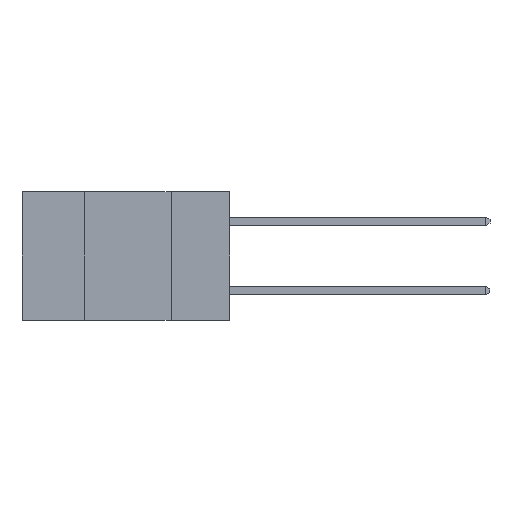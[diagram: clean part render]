
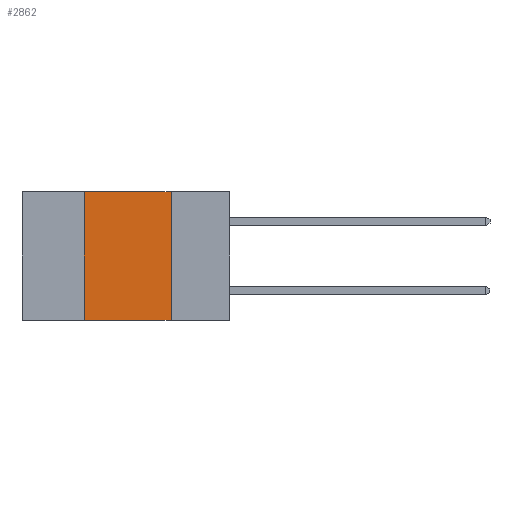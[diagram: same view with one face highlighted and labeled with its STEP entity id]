
A CAD part, left-side view. The second image highlights one B-rep face of the part: STEP entity #2862.
In plain terms, the highlighted planar face has unit normal (-1, 0, 0).
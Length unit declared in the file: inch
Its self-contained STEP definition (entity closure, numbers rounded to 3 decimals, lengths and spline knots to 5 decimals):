
#152 = CARTESIAN_POINT ( 'NONE',  ( 0., 0.42, -0.37 ) ) ;
#434 = AXIS2_PLACEMENT_3D ( 'NONE', #6717, #8320, #8428 ) ;
#1531 = CARTESIAN_POINT ( 'NONE',  ( 0., 0.6, 0. ) ) ;
#1927 = CARTESIAN_POINT ( 'NONE',  ( 0., 0.17, -0.37 ) ) ;
#2066 = VERTEX_POINT ( 'NONE', #1927 ) ;
#2510 = VERTEX_POINT ( 'NONE', #152 ) ;
#2635 = ORIENTED_EDGE ( 'NONE', *, *, #4896, .T. ) ;
#2862 = ADVANCED_FACE ( 'NONE', ( #8145 ), #3602, .F. ) ;
#2892 = ORIENTED_EDGE ( 'NONE', *, *, #6608, .F. ) ;
#3064 = LINE ( 'NONE', #9237, #8705 ) ;
#3136 = ORIENTED_EDGE ( 'NONE', *, *, #3568, .F. ) ;
#3568 = EDGE_CURVE ( 'NONE', #6041, #6629, #7352, .T. ) ;
#3602 = PLANE ( 'NONE',  #434 ) ;
#3685 = VECTOR ( 'NONE', #8770, 39.37008 ) ;
#3929 = DIRECTION ( 'NONE',  ( 0., -1., 0. ) ) ;
#4471 = EDGE_LOOP ( 'NONE', ( #2892, #3136, #6456, #2635 ) ) ;
#4896 = EDGE_CURVE ( 'NONE', #2510, #2066, #7546, .T. ) ;
#5278 = LINE ( 'NONE', #6050, #8507 ) ;
#5432 = DIRECTION ( 'NONE',  ( 0., 0., 1. ) ) ;
#6041 = VERTEX_POINT ( 'NONE', #7621 ) ;
#6050 = CARTESIAN_POINT ( 'NONE',  ( 0., 0.17, 0. ) ) ;
#6456 = ORIENTED_EDGE ( 'NONE', *, *, #6627, .F. ) ;
#6608 = EDGE_CURVE ( 'NONE', #6629, #2066, #5278, .T. ) ;
#6627 = EDGE_CURVE ( 'NONE', #2510, #6041, #3064, .T. ) ;
#6629 = VERTEX_POINT ( 'NONE', #8641 ) ;
#6695 = DIRECTION ( 'NONE',  ( 0., 0., -1. ) ) ;
#6717 = CARTESIAN_POINT ( 'NONE',  ( 0., 0.6, 0. ) ) ;
#7352 = LINE ( 'NONE', #1531, #3685 ) ;
#7546 = LINE ( 'NONE', #7665, #8795 ) ;
#7621 = CARTESIAN_POINT ( 'NONE',  ( 0., 0.42, 0. ) ) ;
#7665 = CARTESIAN_POINT ( 'NONE',  ( 0., 0.6, -0.37 ) ) ;
#8145 = FACE_OUTER_BOUND ( 'NONE', #4471, .T. ) ;
#8320 = DIRECTION ( 'NONE',  ( 1., 0., 0. ) ) ;
#8428 = DIRECTION ( 'NONE',  ( 0., 0., -1. ) ) ;
#8507 = VECTOR ( 'NONE', #6695, 39.37008 ) ;
#8641 = CARTESIAN_POINT ( 'NONE',  ( 0., 0.17, 0. ) ) ;
#8705 = VECTOR ( 'NONE', #5432, 39.37008 ) ;
#8770 = DIRECTION ( 'NONE',  ( 0., -1., 0. ) ) ;
#8795 = VECTOR ( 'NONE', #3929, 39.37008 ) ;
#9237 = CARTESIAN_POINT ( 'NONE',  ( 0., 0.42, 0. ) ) ;
